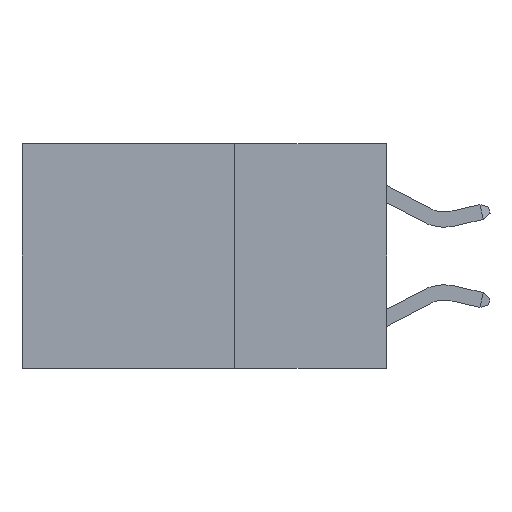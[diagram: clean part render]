
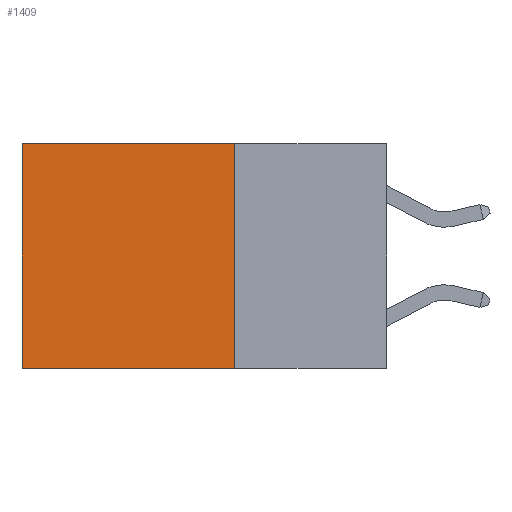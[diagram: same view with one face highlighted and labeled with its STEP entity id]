
A CAD part, left-side view. The second image highlights one B-rep face of the part: STEP entity #1409.
In plain terms, the highlighted planar face has unit normal (-1, 0, 0).
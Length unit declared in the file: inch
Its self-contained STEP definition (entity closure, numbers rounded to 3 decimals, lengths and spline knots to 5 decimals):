
#95 = CARTESIAN_POINT ( 'NONE',  ( 0.2625, 0.25, 0. ) ) ;
#208 = ORIENTED_EDGE ( 'NONE', *, *, #9428, .T. ) ;
#1169 = VECTOR ( 'NONE', #9397, 39.37008 ) ;
#1409 = ADVANCED_FACE ( 'NONE', ( #3818 ), #4116, .F. ) ;
#1924 = AXIS2_PLACEMENT_3D ( 'NONE', #12412, #6504, #6700 ) ;
#1953 = EDGE_CURVE ( 'NONE', #11680, #6291, #14555, .T. ) ;
#2606 = DIRECTION ( 'NONE',  ( 0., 1., 0. ) ) ;
#2865 = CARTESIAN_POINT ( 'NONE',  ( 0.2625, 0.25, -0.37 ) ) ;
#3140 = CARTESIAN_POINT ( 'NONE',  ( 0.2625, 0.6, -0.37 ) ) ;
#3818 = FACE_OUTER_BOUND ( 'NONE', #7506, .T. ) ;
#4116 = PLANE ( 'NONE',  #1924 ) ;
#4802 = CARTESIAN_POINT ( 'NONE',  ( 0.2625, 0.6, 0. ) ) ;
#5356 = LINE ( 'NONE', #10370, #5912 ) ;
#5480 = CARTESIAN_POINT ( 'NONE',  ( 0.2625, 0.25, 0. ) ) ;
#5912 = VECTOR ( 'NONE', #10617, 39.37008 ) ;
#6149 = CARTESIAN_POINT ( 'NONE',  ( 0.2625, 0.25, -0.37 ) ) ;
#6291 = VERTEX_POINT ( 'NONE', #2865 ) ;
#6472 = VECTOR ( 'NONE', #2606, 39.37008 ) ;
#6504 = DIRECTION ( 'NONE',  ( 1., 0., 0. ) ) ;
#6700 = DIRECTION ( 'NONE',  ( 0., 0., -1. ) ) ;
#6757 = DIRECTION ( 'NONE',  ( 0., 0., -1. ) ) ;
#6822 = VERTEX_POINT ( 'NONE', #3140 ) ;
#7045 = VERTEX_POINT ( 'NONE', #4802 ) ;
#7350 = EDGE_CURVE ( 'NONE', #11680, #7045, #5356, .T. ) ;
#7506 = EDGE_LOOP ( 'NONE', ( #208, #11387, #8145, #12705 ) ) ;
#7754 = LINE ( 'NONE', #6149, #6472 ) ;
#8060 = VECTOR ( 'NONE', #6757, 39.37008 ) ;
#8145 = ORIENTED_EDGE ( 'NONE', *, *, #1953, .F. ) ;
#9397 = DIRECTION ( 'NONE',  ( 0., 0., -1. ) ) ;
#9428 = EDGE_CURVE ( 'NONE', #7045, #6822, #11248, .T. ) ;
#10370 = CARTESIAN_POINT ( 'NONE',  ( 0.2625, 0.25, 0. ) ) ;
#10617 = DIRECTION ( 'NONE',  ( 0., 1., 0. ) ) ;
#11248 = LINE ( 'NONE', #15376, #1169 ) ;
#11387 = ORIENTED_EDGE ( 'NONE', *, *, #13338, .F. ) ;
#11680 = VERTEX_POINT ( 'NONE', #95 ) ;
#12412 = CARTESIAN_POINT ( 'NONE',  ( 0.2625, 0.25, 0. ) ) ;
#12705 = ORIENTED_EDGE ( 'NONE', *, *, #7350, .T. ) ;
#13338 = EDGE_CURVE ( 'NONE', #6291, #6822, #7754, .T. ) ;
#14555 = LINE ( 'NONE', #5480, #8060 ) ;
#15376 = CARTESIAN_POINT ( 'NONE',  ( 0.2625, 0.6, 0. ) ) ;
